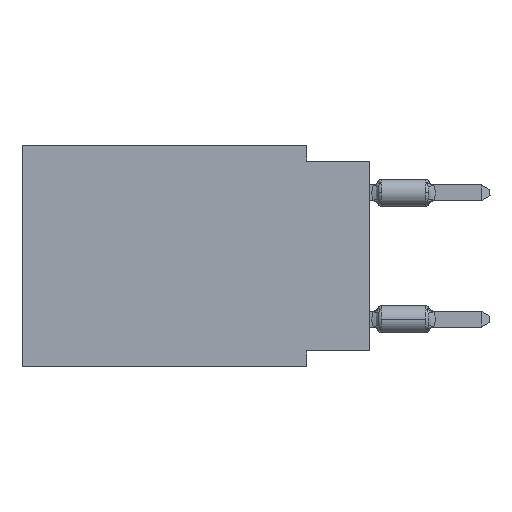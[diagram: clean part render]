
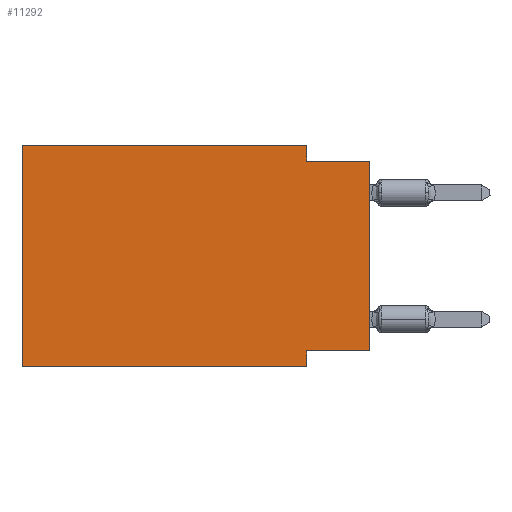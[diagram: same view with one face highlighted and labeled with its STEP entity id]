
A CAD part, left-side view. The second image highlights one B-rep face of the part: STEP entity #11292.
In plain terms, the highlighted planar face has unit normal (-1, 0, 0).
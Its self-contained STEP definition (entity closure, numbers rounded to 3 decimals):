
#487 = LINE ( 'NONE', #8566, #18148 ) ;
#677 = LINE ( 'NONE', #10884, #5637 ) ;
#770 = CARTESIAN_POINT ( 'NONE',  ( 0., 2.54, 0. ) ) ;
#911 = DIRECTION ( 'NONE',  ( 0., 0., -1. ) ) ;
#1304 = PLANE ( 'NONE',  #5512 ) ;
#1312 = DIRECTION ( 'NONE',  ( 0., 0., 1. ) ) ;
#1461 = VECTOR ( 'NONE', #10366, 1000. ) ;
#1547 = CARTESIAN_POINT ( 'NONE',  ( 0., 13.97, 0. ) ) ;
#1617 = EDGE_CURVE ( 'NONE', #17991, #21388, #4354, .T. ) ;
#2014 = VECTOR ( 'NONE', #23695, 1000. ) ;
#2195 = ORIENTED_EDGE ( 'NONE', *, *, #1617, .F. ) ;
#2394 = VECTOR ( 'NONE', #20756, 1000. ) ;
#2635 = DIRECTION ( 'NONE',  ( 0., 0., -1. ) ) ;
#2987 = EDGE_CURVE ( 'NONE', #16398, #11500, #677, .T. ) ;
#3686 = CARTESIAN_POINT ( 'NONE',  ( 0., 13.97, -8.89 ) ) ;
#4247 = CARTESIAN_POINT ( 'NONE',  ( 0., 13.97, 0. ) ) ;
#4271 = CARTESIAN_POINT ( 'NONE',  ( 0., 13.97, -8.89 ) ) ;
#4354 = LINE ( 'NONE', #24720, #25497 ) ;
#5073 = EDGE_CURVE ( 'NONE', #11707, #16398, #12702, .T. ) ;
#5512 = AXIS2_PLACEMENT_3D ( 'NONE', #11376, #14483, #911 ) ;
#5637 = VECTOR ( 'NONE', #17105, 1000. ) ;
#5971 = EDGE_CURVE ( 'NONE', #11473, #21411, #17763, .T. ) ;
#8313 = CARTESIAN_POINT ( 'NONE',  ( 0., 0., -0.635 ) ) ;
#8566 = CARTESIAN_POINT ( 'NONE',  ( 0., 0., -8.255 ) ) ;
#8700 = CARTESIAN_POINT ( 'NONE',  ( 0., 2.54, 0. ) ) ;
#9164 = EDGE_CURVE ( 'NONE', #10901, #17991, #487, .T. ) ;
#10366 = DIRECTION ( 'NONE',  ( 0., -1., 0. ) ) ;
#10884 = CARTESIAN_POINT ( 'NONE',  ( 0., 0., -0.635 ) ) ;
#10901 = VERTEX_POINT ( 'NONE', #11438 ) ;
#11292 = ADVANCED_FACE ( 'NONE', ( #21414 ), #1304, .F. ) ;
#11376 = CARTESIAN_POINT ( 'NONE',  ( 0., 13.97, 0. ) ) ;
#11438 = CARTESIAN_POINT ( 'NONE',  ( 0., 0., -8.255 ) ) ;
#11473 = VERTEX_POINT ( 'NONE', #3686 ) ;
#11500 = VERTEX_POINT ( 'NONE', #8313 ) ;
#11657 = CARTESIAN_POINT ( 'NONE',  ( 0., 13.97, 0. ) ) ;
#11707 = VERTEX_POINT ( 'NONE', #8700 ) ;
#12061 = CARTESIAN_POINT ( 'NONE',  ( 0., 2.54, -8.255 ) ) ;
#12385 = ORIENTED_EDGE ( 'NONE', *, *, #5073, .F. ) ;
#12702 = LINE ( 'NONE', #770, #2394 ) ;
#13951 = ORIENTED_EDGE ( 'NONE', *, *, #22939, .T. ) ;
#13996 = ORIENTED_EDGE ( 'NONE', *, *, #2987, .F. ) ;
#14309 = EDGE_CURVE ( 'NONE', #21411, #11707, #22054, .T. ) ;
#14483 = DIRECTION ( 'NONE',  ( 1., 0., 0. ) ) ;
#15588 = ORIENTED_EDGE ( 'NONE', *, *, #5971, .F. ) ;
#15873 = DIRECTION ( 'NONE',  ( 0., -1., 0. ) ) ;
#16398 = VERTEX_POINT ( 'NONE', #18659 ) ;
#17105 = DIRECTION ( 'NONE',  ( 0., -1., 0. ) ) ;
#17335 = EDGE_LOOP ( 'NONE', ( #13951, #13996, #12385, #24035, #15588, #22430, #2195, #20927 ) ) ;
#17763 = LINE ( 'NONE', #11657, #2014 ) ;
#17991 = VERTEX_POINT ( 'NONE', #12061 ) ;
#18148 = VECTOR ( 'NONE', #24693, 1000. ) ;
#18659 = CARTESIAN_POINT ( 'NONE',  ( 0., 2.54, -0.635 ) ) ;
#18919 = EDGE_CURVE ( 'NONE', #11473, #21388, #24127, .T. ) ;
#19451 = CARTESIAN_POINT ( 'NONE',  ( 0., 0., 0. ) ) ;
#19994 = VECTOR ( 'NONE', #15873, 1000. ) ;
#20756 = DIRECTION ( 'NONE',  ( 0., 0., -1. ) ) ;
#20927 = ORIENTED_EDGE ( 'NONE', *, *, #9164, .F. ) ;
#21388 = VERTEX_POINT ( 'NONE', #24100 ) ;
#21411 = VERTEX_POINT ( 'NONE', #4247 ) ;
#21414 = FACE_OUTER_BOUND ( 'NONE', #17335, .T. ) ;
#21892 = VECTOR ( 'NONE', #1312, 1000. ) ;
#22054 = LINE ( 'NONE', #1547, #19994 ) ;
#22430 = ORIENTED_EDGE ( 'NONE', *, *, #18919, .T. ) ;
#22939 = EDGE_CURVE ( 'NONE', #10901, #11500, #23280, .T. ) ;
#23280 = LINE ( 'NONE', #19451, #21892 ) ;
#23695 = DIRECTION ( 'NONE',  ( 0., 0., 1. ) ) ;
#24035 = ORIENTED_EDGE ( 'NONE', *, *, #14309, .F. ) ;
#24100 = CARTESIAN_POINT ( 'NONE',  ( 0., 2.54, -8.89 ) ) ;
#24127 = LINE ( 'NONE', #4271, #1461 ) ;
#24693 = DIRECTION ( 'NONE',  ( 0., 1., 0. ) ) ;
#24720 = CARTESIAN_POINT ( 'NONE',  ( 0., 2.54, -8.89 ) ) ;
#25497 = VECTOR ( 'NONE', #2635, 1000. ) ;
